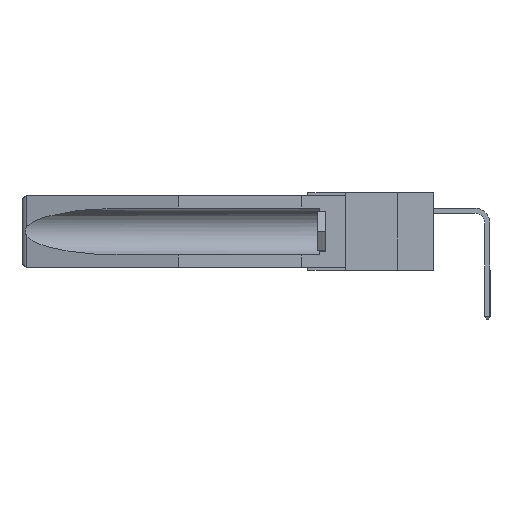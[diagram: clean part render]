
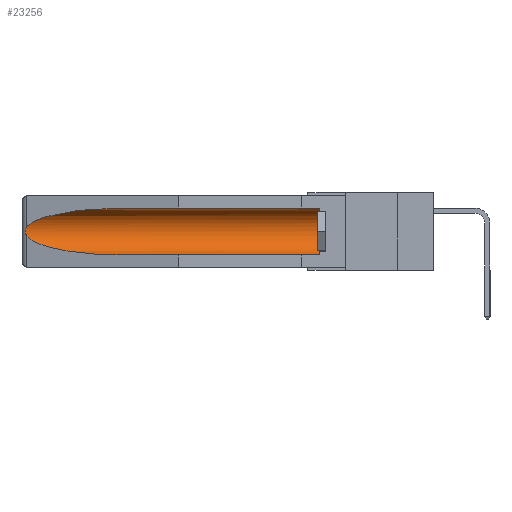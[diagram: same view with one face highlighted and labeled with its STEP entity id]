
A CAD part, left-side view. The second image highlights one B-rep face of the part: STEP entity #23256.
In plain terms, the highlighted cylindrical face has radius 2.857 mm (diameter 5.715 mm), a partial arc.
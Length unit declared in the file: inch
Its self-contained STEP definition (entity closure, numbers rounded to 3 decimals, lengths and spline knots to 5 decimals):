
#75 = CARTESIAN_POINT ( 'NONE',  ( 0.2673, 1.5327, -0.16383 ) ) ;
#393 =( BOUNDED_CURVE ( )  B_SPLINE_CURVE ( 3, ( #17269, #2692, #5133, #19389 ),
 .UNSPECIFIED., .F., .F. ) 
 B_SPLINE_CURVE_WITH_KNOTS ( ( 4, 4 ),
 ( 0.1948, 1.5708 ),
 .UNSPECIFIED. ) 
 CURVE ( )  GEOMETRIC_REPRESENTATION_ITEM ( )  RATIONAL_B_SPLINE_CURVE ( ( 1., 0.848, 0.848, 1. ) ) 
 REPRESENTATION_ITEM ( '' )  );
#430 = EDGE_LOOP ( 'NONE', ( #31456, #26365, #3095, #1501, #30595, #20462 ) ) ;
#1058 = CARTESIAN_POINT ( 'NONE',  ( 0.155, 0.126, -0.059 ) ) ;
#1490 = LINE ( 'NONE', #11009, #3372 ) ;
#1501 = ORIENTED_EDGE ( 'NONE', *, *, #4769, .F. ) ;
#1548 = DIRECTION ( 'NONE',  ( 0., 0., 1. ) ) ;
#1663 = EDGE_CURVE ( 'NONE', #18184, #29219, #28182, .T. ) ;
#1670 = DIRECTION ( 'NONE',  ( 0., 1., 0. ) ) ;
#2516 = CARTESIAN_POINT ( 'NONE',  ( 0.26537, 1.52718, -0.19328 ) ) ;
#2692 = CARTESIAN_POINT ( 'NONE',  ( 0.25451, 1.48313, -0.24835 ) ) ;
#2818 = CARTESIAN_POINT ( 'NONE',  ( 0.2673, 1.53269, -0.17917 ) ) ;
#3095 = ORIENTED_EDGE ( 'NONE', *, *, #13095, .T. ) ;
#3372 = VECTOR ( 'NONE', #30608, 39.37008 ) ;
#3905 = VECTOR ( 'NONE', #21765, 39.37008 ) ;
#4769 = EDGE_CURVE ( 'NONE', #8924, #26209, #19898, .T. ) ;
#4949 = CARTESIAN_POINT ( 'NONE',  ( 0.26655, 1.53094, -0.18657 ) ) ;
#5133 = CARTESIAN_POINT ( 'NONE',  ( 0.21114, 1.30732, -0.284 ) ) ;
#6043 =( BOUNDED_CURVE ( )  B_SPLINE_CURVE ( 3, ( #25516, #22989, #11098, #27652 ),
 .UNSPECIFIED., .F., .F. ) 
 B_SPLINE_CURVE_WITH_KNOTS ( ( 4, 4 ),
 ( 4.71239, 6.08839 ),
 .UNSPECIFIED. ) 
 CURVE ( )  GEOMETRIC_REPRESENTATION_ITEM ( )  RATIONAL_B_SPLINE_CURVE ( ( 1., 0.848, 0.848, 1. ) ) 
 REPRESENTATION_ITEM ( '' )  );
#7045 = CARTESIAN_POINT ( 'NONE',  ( 0.155, 1.07973, -0.284 ) ) ;
#7618 = CARTESIAN_POINT ( 'NONE',  ( 0.26597, 1.52961, -0.15275 ) ) ;
#7825 = CARTESIAN_POINT ( 'NONE',  ( 0.26597, 1.5296, -0.19026 ) ) ;
#8924 = VERTEX_POINT ( 'NONE', #23182 ) ;
#9105 = AXIS2_PLACEMENT_3D ( 'NONE', #11243, #1670, #20860 ) ;
#9831 = CARTESIAN_POINT ( 'NONE',  ( 0.26537, 1.52718, -0.14972 ) ) ;
#11009 = CARTESIAN_POINT ( 'NONE',  ( 0.155, -0.30754, -0.059 ) ) ;
#11098 = CARTESIAN_POINT ( 'NONE',  ( 0.25451, 1.48313, -0.09465 ) ) ;
#11243 = CARTESIAN_POINT ( 'NONE',  ( 0.155, -0.30754, -0.1715 ) ) ;
#11536 = EDGE_CURVE ( 'NONE', #20358, #18184, #6043, .T. ) ;
#12796 = EDGE_CURVE ( 'NONE', #8924, #18530, #15013, .T. ) ;
#13095 = EDGE_CURVE ( 'NONE', #29219, #26209, #393, .T. ) ;
#14173 = FACE_OUTER_BOUND ( 'NONE', #430, .T. ) ;
#14302 = CARTESIAN_POINT ( 'NONE',  ( 0.26537, 1.52718, -0.19328 ) ) ;
#14580 = CYLINDRICAL_SURFACE ( 'NONE', #9105, 0.1125 ) ;
#14659 = CARTESIAN_POINT ( 'NONE',  ( 0.2675, 1.53308, -0.16763 ) ) ;
#15013 = CIRCLE ( 'NONE', #31172, 0.1125 ) ;
#16211 = DIRECTION ( 'NONE',  ( 0., -1., 0. ) ) ;
#17191 = CARTESIAN_POINT ( 'NONE',  ( 0.2675, 1.53308, -0.17534 ) ) ;
#17269 = CARTESIAN_POINT ( 'NONE',  ( 0.26537, 1.52718, -0.19328 ) ) ;
#18184 = VERTEX_POINT ( 'NONE', #21087 ) ;
#18530 = VERTEX_POINT ( 'NONE', #1058 ) ;
#19235 = EDGE_CURVE ( 'NONE', #18530, #20358, #1490, .T. ) ;
#19389 = CARTESIAN_POINT ( 'NONE',  ( 0.155, 1.07973, -0.284 ) ) ;
#19898 = LINE ( 'NONE', #31284, #3905 ) ;
#20358 = VERTEX_POINT ( 'NONE', #27692 ) ;
#20462 = ORIENTED_EDGE ( 'NONE', *, *, #19235, .T. ) ;
#20860 = DIRECTION ( 'NONE',  ( 0., 0., 1. ) ) ;
#21087 = CARTESIAN_POINT ( 'NONE',  ( 0.26537, 1.52718, -0.14972 ) ) ;
#21765 = DIRECTION ( 'NONE',  ( 0., 1., 0. ) ) ;
#22989 = CARTESIAN_POINT ( 'NONE',  ( 0.21114, 1.30732, -0.059 ) ) ;
#23182 = CARTESIAN_POINT ( 'NONE',  ( 0.155, 0.126, -0.284 ) ) ;
#23256 = ADVANCED_FACE ( 'NONE', ( #14173 ), #14580, .F. ) ;
#25516 = CARTESIAN_POINT ( 'NONE',  ( 0.155, 1.07973, -0.059 ) ) ;
#26042 = CARTESIAN_POINT ( 'NONE',  ( 0.155, 0.126, -0.1715 ) ) ;
#26209 = VERTEX_POINT ( 'NONE', #7045 ) ;
#26365 = ORIENTED_EDGE ( 'NONE', *, *, #1663, .T. ) ;
#26812 = CARTESIAN_POINT ( 'NONE',  ( 0.26654, 1.53092, -0.15636 ) ) ;
#27652 = CARTESIAN_POINT ( 'NONE',  ( 0.26537, 1.52718, -0.14972 ) ) ;
#27692 = CARTESIAN_POINT ( 'NONE',  ( 0.155, 1.07973, -0.059 ) ) ;
#28182 = B_SPLINE_CURVE_WITH_KNOTS ( 'NONE', 3,
 ( #9831, #7618, #26812, #75, #14659, #17191, #2818, #4949, #7825, #2516 ),
 .UNSPECIFIED., .F., .F.,
 ( 4, 2, 2, 2, 4 ),
 ( 0., 0.00029, 0.00058, 0.00087, 0.00117 ),
 .UNSPECIFIED. ) ;
#29219 = VERTEX_POINT ( 'NONE', #14302 ) ;
#30595 = ORIENTED_EDGE ( 'NONE', *, *, #12796, .T. ) ;
#30608 = DIRECTION ( 'NONE',  ( 0., 1., 0. ) ) ;
#31172 = AXIS2_PLACEMENT_3D ( 'NONE', #26042, #16211, #1548 ) ;
#31284 = CARTESIAN_POINT ( 'NONE',  ( 0.155, -0.30754, -0.284 ) ) ;
#31456 = ORIENTED_EDGE ( 'NONE', *, *, #11536, .T. ) ;
